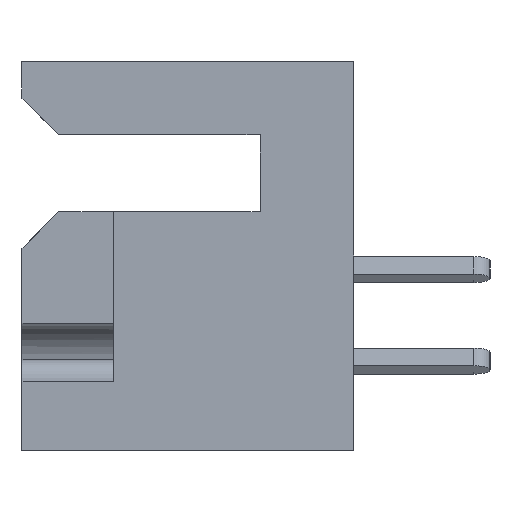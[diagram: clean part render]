
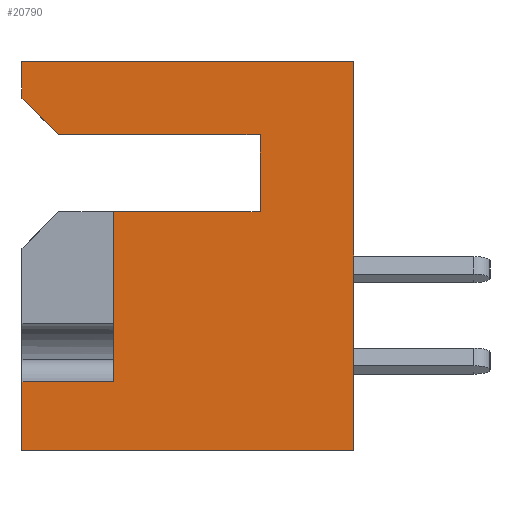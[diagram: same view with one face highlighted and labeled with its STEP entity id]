
A CAD part, left-side view. The second image highlights one B-rep face of the part: STEP entity #20790.
In plain terms, the highlighted planar face has unit normal (-1, 0, 0).
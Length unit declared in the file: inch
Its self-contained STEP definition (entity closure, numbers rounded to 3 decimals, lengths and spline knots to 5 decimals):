
#272 = EDGE_CURVE ( 'NONE', #5375, #12966, #8070, .T. ) ;
#528 = LINE ( 'NONE', #8600, #11909 ) ;
#1201 = AXIS2_PLACEMENT_3D ( 'NONE', #3447, #9811, #10090 ) ;
#1562 = VECTOR ( 'NONE', #2158, 39.37008 ) ;
#1648 = ORIENTED_EDGE ( 'NONE', *, *, #3351, .F. ) ;
#1865 = CARTESIAN_POINT ( 'NONE',  ( 0., 0.328, -0.205 ) ) ;
#2088 = CARTESIAN_POINT ( 'NONE',  ( 0., 0.453, 0. ) ) ;
#2158 = DIRECTION ( 'NONE',  ( 0., 0., 1. ) ) ;
#2329 = DIRECTION ( 'NONE',  ( 0., 0., 1. ) ) ;
#2426 = VERTEX_POINT ( 'NONE', #9501 ) ;
#2635 = VECTOR ( 'NONE', #7017, 39.37008 ) ;
#3208 = VECTOR ( 'NONE', #11241, 39.37008 ) ;
#3219 = ORIENTED_EDGE ( 'NONE', *, *, #20355, .T. ) ;
#3351 = EDGE_CURVE ( 'NONE', #13049, #8761, #10665, .T. ) ;
#3447 = CARTESIAN_POINT ( 'NONE',  ( 0., 0.453, 0. ) ) ;
#3475 = CARTESIAN_POINT ( 'NONE',  ( 0., 0.453, -0.05 ) ) ;
#3585 = VERTEX_POINT ( 'NONE', #18782 ) ;
#3675 = CARTESIAN_POINT ( 'NONE',  ( 0., 0.453, 0. ) ) ;
#3775 = VECTOR ( 'NONE', #4889, 39.37008 ) ;
#3882 = LINE ( 'NONE', #19611, #16340 ) ;
#4012 = VECTOR ( 'NONE', #2329, 39.37008 ) ;
#4889 = DIRECTION ( 'NONE',  ( 0., 0., 1. ) ) ;
#5233 = DIRECTION ( 'NONE',  ( 0., -0.707, -0.707 ) ) ;
#5375 = VERTEX_POINT ( 'NONE', #3475 ) ;
#5564 = CARTESIAN_POINT ( 'NONE',  ( 0., 0.128, -0.1 ) ) ;
#5807 = CARTESIAN_POINT ( 'NONE',  ( 0., 0.128, -0.205 ) ) ;
#6067 = FACE_OUTER_BOUND ( 'NONE', #6402, .T. ) ;
#6076 = LINE ( 'NONE', #6651, #7594 ) ;
#6402 = EDGE_LOOP ( 'NONE', ( #6738, #7994, #13934, #17942, #9932, #20298, #3219, #8848, #14798, #9961, #1648 ) ) ;
#6450 = CARTESIAN_POINT ( 'NONE',  ( 0., 0.328, -0.205 ) ) ;
#6651 = CARTESIAN_POINT ( 'NONE',  ( 0., 0.403, -0.1 ) ) ;
#6659 = CARTESIAN_POINT ( 'NONE',  ( 0., 0.403, -0.1 ) ) ;
#6699 = DIRECTION ( 'NONE',  ( 0., 0., 1. ) ) ;
#6738 = ORIENTED_EDGE ( 'NONE', *, *, #13218, .T. ) ;
#6819 = EDGE_CURVE ( 'NONE', #13446, #2426, #3882, .T. ) ;
#7017 = DIRECTION ( 'NONE',  ( 0., 0., 1. ) ) ;
#7098 = CARTESIAN_POINT ( 'NONE',  ( 0., 0.128, -0.1 ) ) ;
#7594 = VECTOR ( 'NONE', #5233, 39.37008 ) ;
#7889 = CARTESIAN_POINT ( 'NONE',  ( 0., 0.128, -0.1 ) ) ;
#7994 = ORIENTED_EDGE ( 'NONE', *, *, #20444, .F. ) ;
#8070 = LINE ( 'NONE', #19648, #3775 ) ;
#8304 = LINE ( 'NONE', #12015, #4012 ) ;
#8445 = LINE ( 'NONE', #20282, #17352 ) ;
#8600 = CARTESIAN_POINT ( 'NONE',  ( 0., 0.328, -0.437 ) ) ;
#8682 = DIRECTION ( 'NONE',  ( 0., 1., 0. ) ) ;
#8761 = VERTEX_POINT ( 'NONE', #6450 ) ;
#8848 = ORIENTED_EDGE ( 'NONE', *, *, #16421, .F. ) ;
#9501 = CARTESIAN_POINT ( 'NONE',  ( 0., 0., -0.531 ) ) ;
#9811 = DIRECTION ( 'NONE',  ( 1., 0., 0. ) ) ;
#9932 = ORIENTED_EDGE ( 'NONE', *, *, #19041, .F. ) ;
#9961 = ORIENTED_EDGE ( 'NONE', *, *, #10262, .T. ) ;
#10090 = DIRECTION ( 'NONE',  ( 0., 0., -1. ) ) ;
#10138 = VECTOR ( 'NONE', #6699, 39.37008 ) ;
#10167 = LINE ( 'NONE', #3675, #15512 ) ;
#10262 = EDGE_CURVE ( 'NONE', #20661, #8761, #8445, .T. ) ;
#10665 = LINE ( 'NONE', #1865, #10138 ) ;
#10803 = EDGE_CURVE ( 'NONE', #20661, #16189, #13511, .T. ) ;
#11241 = DIRECTION ( 'NONE',  ( 0., 1., 0. ) ) ;
#11338 = CARTESIAN_POINT ( 'NONE',  ( 0., 0.328, -0.437 ) ) ;
#11826 = LINE ( 'NONE', #7889, #3208 ) ;
#11909 = VECTOR ( 'NONE', #8682, 39.37008 ) ;
#12015 = CARTESIAN_POINT ( 'NONE',  ( 0., 0., 0. ) ) ;
#12966 = VERTEX_POINT ( 'NONE', #15834 ) ;
#13049 = VERTEX_POINT ( 'NONE', #11338 ) ;
#13129 = DIRECTION ( 'NONE',  ( 0., -1., 0. ) ) ;
#13218 = EDGE_CURVE ( 'NONE', #13049, #3585, #528, .T. ) ;
#13375 = DIRECTION ( 'NONE',  ( 0., -1., 0. ) ) ;
#13446 = VERTEX_POINT ( 'NONE', #14219 ) ;
#13511 = LINE ( 'NONE', #7098, #2635 ) ;
#13846 = EDGE_CURVE ( 'NONE', #2426, #17253, #8304, .T. ) ;
#13934 = ORIENTED_EDGE ( 'NONE', *, *, #6819, .T. ) ;
#14219 = CARTESIAN_POINT ( 'NONE',  ( 0., 0.453, -0.531 ) ) ;
#14798 = ORIENTED_EDGE ( 'NONE', *, *, #10803, .F. ) ;
#14855 = CARTESIAN_POINT ( 'NONE',  ( 0., 0., 0. ) ) ;
#15226 = DIRECTION ( 'NONE',  ( 0., 1., 0. ) ) ;
#15512 = VECTOR ( 'NONE', #13375, 39.37008 ) ;
#15834 = CARTESIAN_POINT ( 'NONE',  ( 0., 0.453, 0. ) ) ;
#16189 = VERTEX_POINT ( 'NONE', #5564 ) ;
#16340 = VECTOR ( 'NONE', #13129, 39.37008 ) ;
#16421 = EDGE_CURVE ( 'NONE', #16189, #16566, #11826, .T. ) ;
#16566 = VERTEX_POINT ( 'NONE', #6659 ) ;
#17253 = VERTEX_POINT ( 'NONE', #14855 ) ;
#17352 = VECTOR ( 'NONE', #15226, 39.37008 ) ;
#17907 = PLANE ( 'NONE',  #1201 ) ;
#17942 = ORIENTED_EDGE ( 'NONE', *, *, #13846, .T. ) ;
#18521 = LINE ( 'NONE', #2088, #1562 ) ;
#18782 = CARTESIAN_POINT ( 'NONE',  ( 0., 0.453, -0.437 ) ) ;
#19041 = EDGE_CURVE ( 'NONE', #12966, #17253, #10167, .T. ) ;
#19611 = CARTESIAN_POINT ( 'NONE',  ( 0., 0.453, -0.531 ) ) ;
#19648 = CARTESIAN_POINT ( 'NONE',  ( 0., 0.453, 0. ) ) ;
#20282 = CARTESIAN_POINT ( 'NONE',  ( 0., 0.128, -0.205 ) ) ;
#20298 = ORIENTED_EDGE ( 'NONE', *, *, #272, .F. ) ;
#20355 = EDGE_CURVE ( 'NONE', #5375, #16566, #6076, .T. ) ;
#20444 = EDGE_CURVE ( 'NONE', #13446, #3585, #18521, .T. ) ;
#20661 = VERTEX_POINT ( 'NONE', #5807 ) ;
#20790 = ADVANCED_FACE ( 'NONE', ( #6067 ), #17907, .F. ) ;
